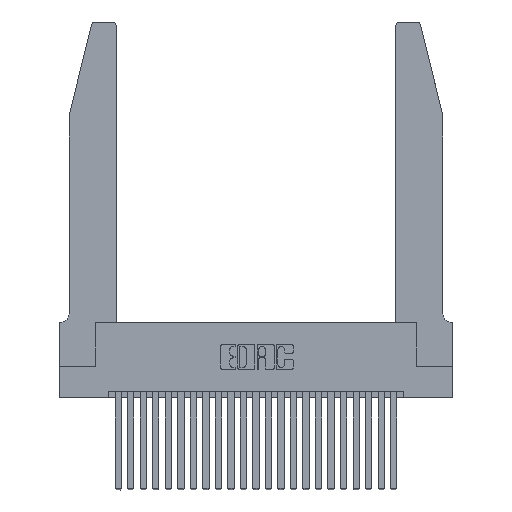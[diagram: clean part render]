
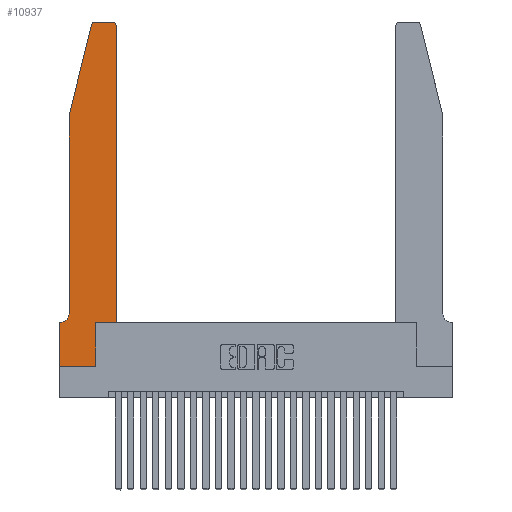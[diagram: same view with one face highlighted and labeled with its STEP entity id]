
A CAD part, top view. The second image highlights one B-rep face of the part: STEP entity #10937.
In plain terms, the highlighted planar face has unit normal (0, 0, 1).
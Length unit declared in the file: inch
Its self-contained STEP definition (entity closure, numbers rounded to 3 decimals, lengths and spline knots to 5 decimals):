
#3 = ORIENTED_EDGE ( 'NONE', *, *, #9728, .T. ) ;
#150 = CARTESIAN_POINT ( 'NONE',  ( 0.2605, 2.75, 0.37 ) ) ;
#926 = CARTESIAN_POINT ( 'NONE',  ( 0.25487, 2.72718, 0.37 ) ) ;
#1028 = DIRECTION ( 'NONE',  ( 0., 1., 0. ) ) ;
#1056 = DIRECTION ( 'NONE',  ( 1., 0., 0. ) ) ;
#1183 = VECTOR ( 'NONE', #6262, 39.37008 ) ;
#1382 = CARTESIAN_POINT ( 'NONE',  ( 0.2865, 0.35, 0.37 ) ) ;
#1425 = AXIS2_PLACEMENT_3D ( 'NONE', #10979, #18685, #7043 ) ;
#1705 = VECTOR ( 'NONE', #23554, 39.37008 ) ;
#1840 = EDGE_CURVE ( 'NONE', #14943, #14656, #6284, .T. ) ;
#2268 = CARTESIAN_POINT ( 'NONE',  ( 0.4505, 0.35, 0.37 ) ) ;
#2407 = CARTESIAN_POINT ( 'NONE',  ( 0.0755, 2., 0.37 ) ) ;
#2498 = CARTESIAN_POINT ( 'NONE',  ( 0.0055, 0.35, 0.37 ) ) ;
#2845 = ORIENTED_EDGE ( 'NONE', *, *, #12847, .T. ) ;
#3169 = EDGE_CURVE ( 'NONE', #10162, #14943, #17102, .T. ) ;
#3217 = ORIENTED_EDGE ( 'NONE', *, *, #16434, .T. ) ;
#3478 = CIRCLE ( 'NONE', #22150, 0.03 ) ;
#3914 = EDGE_CURVE ( 'NONE', #14659, #24120, #3478, .T. ) ;
#3962 = DIRECTION ( 'NONE',  ( 0., 0., 1. ) ) ;
#4057 = CARTESIAN_POINT ( 'NONE',  ( 0.2865, 0., 0.37 ) ) ;
#4158 = LINE ( 'NONE', #2268, #1705 ) ;
#4647 = ORIENTED_EDGE ( 'NONE', *, *, #13324, .T. ) ;
#4701 = VECTOR ( 'NONE', #4894, 39.37008 ) ;
#4894 = DIRECTION ( 'NONE',  ( 0., -1., 0. ) ) ;
#5478 = ORIENTED_EDGE ( 'NONE', *, *, #3914, .T. ) ;
#5894 = LINE ( 'NONE', #23662, #8636 ) ;
#6262 = DIRECTION ( 'NONE',  ( -1., 0., 0. ) ) ;
#6284 = CIRCLE ( 'NONE', #7392, 0.07 ) ;
#6293 = CARTESIAN_POINT ( 'NONE',  ( 0.0755, 0.35, 0.37 ) ) ;
#6432 = CARTESIAN_POINT ( 'NONE',  ( 0.4505, 2.72, 0.37 ) ) ;
#6543 = ORIENTED_EDGE ( 'NONE', *, *, #1840, .T. ) ;
#6608 = VECTOR ( 'NONE', #24564, 39.37008 ) ;
#6894 = CARTESIAN_POINT ( 'NONE',  ( 0.4505, 0.35, 0.37 ) ) ;
#6910 = VERTEX_POINT ( 'NONE', #926 ) ;
#7043 = DIRECTION ( 'NONE',  ( 1., 0., 0. ) ) ;
#7392 = AXIS2_PLACEMENT_3D ( 'NONE', #14877, #24716, #10969 ) ;
#8204 = DIRECTION ( 'NONE',  ( -1., 0., 0. ) ) ;
#8636 = VECTOR ( 'NONE', #17970, 39.37008 ) ;
#9028 = VECTOR ( 'NONE', #1028, 39.37008 ) ;
#9134 = PLANE ( 'NONE',  #1425 ) ;
#9246 = DIRECTION ( 'NONE',  ( 1., 0., 0. ) ) ;
#9728 = EDGE_CURVE ( 'NONE', #6910, #10162, #19633, .T. ) ;
#10162 = VERTEX_POINT ( 'NONE', #24481 ) ;
#10256 = EDGE_CURVE ( 'NONE', #12828, #14659, #23242, .T. ) ;
#10439 = EDGE_LOOP ( 'NONE', ( #13300, #21006, #3, #20887, #6543, #22326, #4647, #2845, #13793, #3217, #21311, #5478 ) ) ;
#10937 = ADVANCED_FACE ( 'NONE', ( #19588 ), #9134, .T. ) ;
#10969 = DIRECTION ( 'NONE',  ( -1., 0., 0. ) ) ;
#10979 = CARTESIAN_POINT ( 'NONE',  ( 0., 0.35, 0.37 ) ) ;
#11000 = CARTESIAN_POINT ( 'NONE',  ( 0., 0., 0.37 ) ) ;
#11310 = VERTEX_POINT ( 'NONE', #13010 ) ;
#12275 = EDGE_CURVE ( 'NONE', #24120, #11310, #15353, .T. ) ;
#12477 = CARTESIAN_POINT ( 'NONE',  ( 0.4505, 0.35, 0.37 ) ) ;
#12828 = VERTEX_POINT ( 'NONE', #6894 ) ;
#12847 = EDGE_CURVE ( 'NONE', #18821, #23076, #14050, .T. ) ;
#13010 = CARTESIAN_POINT ( 'NONE',  ( 0.284, 2.75, 0.37 ) ) ;
#13169 = CARTESIAN_POINT ( 'NONE',  ( 0.0755, 2., 0.37 ) ) ;
#13300 = ORIENTED_EDGE ( 'NONE', *, *, #12275, .T. ) ;
#13324 = EDGE_CURVE ( 'NONE', #16567, #18821, #5894, .T. ) ;
#13793 = ORIENTED_EDGE ( 'NONE', *, *, #25015, .T. ) ;
#14050 = LINE ( 'NONE', #11000, #19213 ) ;
#14323 = AXIS2_PLACEMENT_3D ( 'NONE', #20727, #14817, #1056 ) ;
#14656 = VERTEX_POINT ( 'NONE', #2498 ) ;
#14659 = VERTEX_POINT ( 'NONE', #6432 ) ;
#14764 = EDGE_CURVE ( 'NONE', #14656, #16567, #19377, .T. ) ;
#14817 = DIRECTION ( 'NONE',  ( 0., 0., 1. ) ) ;
#14834 = VECTOR ( 'NONE', #24784, 39.37008 ) ;
#14877 = CARTESIAN_POINT ( 'NONE',  ( 0.0055, 0.42, 0.37 ) ) ;
#14943 = VERTEX_POINT ( 'NONE', #21425 ) ;
#15353 = LINE ( 'NONE', #150, #25071 ) ;
#15496 = CARTESIAN_POINT ( 'NONE',  ( 0.4205, 2.72, 0.37 ) ) ;
#16434 = EDGE_CURVE ( 'NONE', #18757, #12828, #4158, .T. ) ;
#16567 = VERTEX_POINT ( 'NONE', #18663 ) ;
#17102 = LINE ( 'NONE', #2407, #4701 ) ;
#17665 = DIRECTION ( 'NONE',  ( 1., 0., 0. ) ) ;
#17970 = DIRECTION ( 'NONE',  ( 0., -1., 0. ) ) ;
#18663 = CARTESIAN_POINT ( 'NONE',  ( 0., 0.35, 0.37 ) ) ;
#18685 = DIRECTION ( 'NONE',  ( 0., 0., 1. ) ) ;
#18757 = VERTEX_POINT ( 'NONE', #22855 ) ;
#18821 = VERTEX_POINT ( 'NONE', #19612 ) ;
#19213 = VECTOR ( 'NONE', #9246, 39.37008 ) ;
#19377 = LINE ( 'NONE', #6293, #1183 ) ;
#19588 = FACE_OUTER_BOUND ( 'NONE', #10439, .T. ) ;
#19612 = CARTESIAN_POINT ( 'NONE',  ( 0., 0., 0.37 ) ) ;
#19633 = LINE ( 'NONE', #13169, #14834 ) ;
#20727 = CARTESIAN_POINT ( 'NONE',  ( 0.284, 2.72, 0.37 ) ) ;
#20887 = ORIENTED_EDGE ( 'NONE', *, *, #3169, .T. ) ;
#21006 = ORIENTED_EDGE ( 'NONE', *, *, #23375, .T. ) ;
#21311 = ORIENTED_EDGE ( 'NONE', *, *, #10256, .T. ) ;
#21425 = CARTESIAN_POINT ( 'NONE',  ( 0.0755, 0.42, 0.37 ) ) ;
#22150 = AXIS2_PLACEMENT_3D ( 'NONE', #15496, #3962, #17665 ) ;
#22326 = ORIENTED_EDGE ( 'NONE', *, *, #14764, .T. ) ;
#22855 = CARTESIAN_POINT ( 'NONE',  ( 0.2865, 0.35, 0.37 ) ) ;
#23076 = VERTEX_POINT ( 'NONE', #4057 ) ;
#23242 = LINE ( 'NONE', #12477, #9028 ) ;
#23375 = EDGE_CURVE ( 'NONE', #11310, #6910, #24532, .T. ) ;
#23554 = DIRECTION ( 'NONE',  ( 1., 0., 0. ) ) ;
#23662 = CARTESIAN_POINT ( 'NONE',  ( 0., 0., 0.37 ) ) ;
#24120 = VERTEX_POINT ( 'NONE', #24961 ) ;
#24481 = CARTESIAN_POINT ( 'NONE',  ( 0.0755, 2., 0.37 ) ) ;
#24532 = CIRCLE ( 'NONE', #14323, 0.03 ) ;
#24564 = DIRECTION ( 'NONE',  ( 0., 1., 0. ) ) ;
#24716 = DIRECTION ( 'NONE',  ( 0., 0., -1. ) ) ;
#24784 = DIRECTION ( 'NONE',  ( -0.239, -0.971, 0. ) ) ;
#24961 = CARTESIAN_POINT ( 'NONE',  ( 0.4205, 2.75, 0.37 ) ) ;
#25015 = EDGE_CURVE ( 'NONE', #23076, #18757, #25111, .T. ) ;
#25071 = VECTOR ( 'NONE', #8204, 39.37008 ) ;
#25111 = LINE ( 'NONE', #1382, #6608 ) ;
